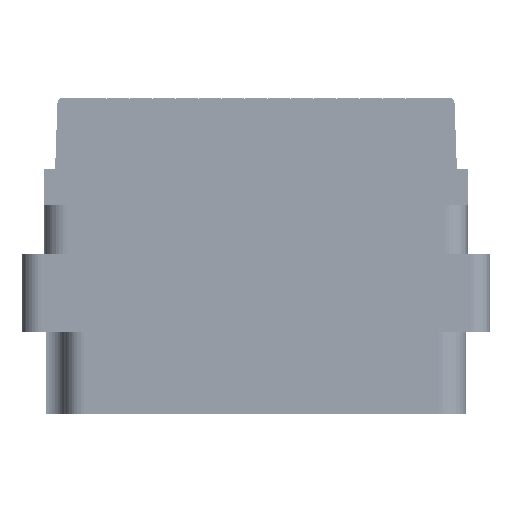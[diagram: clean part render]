
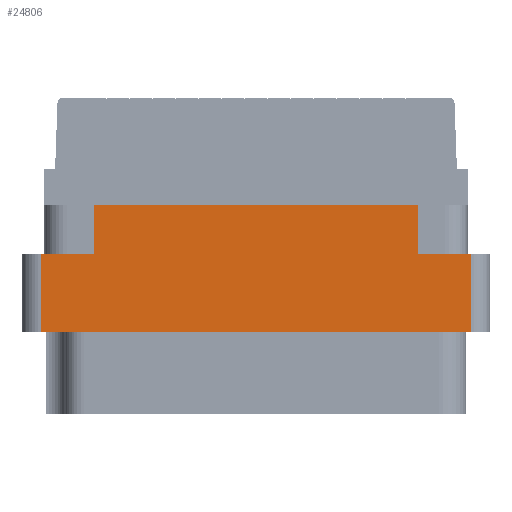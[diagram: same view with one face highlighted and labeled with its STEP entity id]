
A CAD part, left-side view. The second image highlights one B-rep face of the part: STEP entity #24806.
In plain terms, the highlighted planar face has unit normal (-1, 0, 0).
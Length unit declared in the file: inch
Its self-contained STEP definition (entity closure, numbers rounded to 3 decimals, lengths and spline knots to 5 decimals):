
#3618 = VECTOR ( 'NONE', #43353, 39.37008 ) ;
#4624 = LINE ( 'NONE', #77104, #86066 ) ;
#5512 = CARTESIAN_POINT ( 'NONE',  ( -1.375, -0.7005, -0.798 ) ) ;
#7226 = EDGE_CURVE ( 'NONE', #54643, #15740, #71783, .T. ) ;
#7428 = LINE ( 'NONE', #80379, #73741 ) ;
#8888 = AXIS2_PLACEMENT_3D ( 'NONE', #82646, #52647, #38307 ) ;
#11765 = DIRECTION ( 'NONE',  ( 0., 1., 0. ) ) ;
#11824 = VECTOR ( 'NONE', #49394, 39.37008 ) ;
#12568 = ORIENTED_EDGE ( 'NONE', *, *, #87304, .F. ) ;
#12978 = VERTEX_POINT ( 'NONE', #65259 ) ;
#13325 = CARTESIAN_POINT ( 'NONE',  ( -1.375, -0.5285, -0.277 ) ) ;
#13382 = ORIENTED_EDGE ( 'NONE', *, *, #82195, .T. ) ;
#15055 = DIRECTION ( 'NONE',  ( 0., -1., 0. ) ) ;
#15740 = VERTEX_POINT ( 'NONE', #57270 ) ;
#22085 = CARTESIAN_POINT ( 'NONE',  ( -1.375, -0.7005, -0.529 ) ) ;
#22122 = CARTESIAN_POINT ( 'NONE',  ( -1.375, 0.7625, -0.117 ) ) ;
#22387 = EDGE_CURVE ( 'NONE', #30751, #45944, #75189, .T. ) ;
#22728 = CARTESIAN_POINT ( 'NONE',  ( -1.375, 0.7005, -0.529 ) ) ;
#23524 = LINE ( 'NONE', #22122, #43030 ) ;
#24618 = DIRECTION ( 'NONE',  ( 0., 0., -1. ) ) ;
#24674 = VECTOR ( 'NONE', #59379, 39.37008 ) ;
#24806 = ADVANCED_FACE ( 'NONE', ( #39247 ), #74551, .T. ) ;
#29367 = DIRECTION ( 'NONE',  ( 0., 0., 1. ) ) ;
#30264 = LINE ( 'NONE', #60345, #24674 ) ;
#30751 = VERTEX_POINT ( 'NONE', #62207 ) ;
#31819 = VERTEX_POINT ( 'NONE', #46499 ) ;
#34468 = ORIENTED_EDGE ( 'NONE', *, *, #64064, .F. ) ;
#35543 = VERTEX_POINT ( 'NONE', #40451 ) ;
#38307 = DIRECTION ( 'NONE',  ( 0., 0., 1. ) ) ;
#39247 = FACE_OUTER_BOUND ( 'NONE', #76238, .T. ) ;
#40451 = CARTESIAN_POINT ( 'NONE',  ( -1.375, 0.5285, -0.117 ) ) ;
#43030 = VECTOR ( 'NONE', #52158, 39.37008 ) ;
#43353 = DIRECTION ( 'NONE',  ( 0., 0., 1. ) ) ;
#43817 = LINE ( 'NONE', #13325, #3618 ) ;
#45944 = VERTEX_POINT ( 'NONE', #22728 ) ;
#46499 = CARTESIAN_POINT ( 'NONE',  ( -1.375, 0.5285, -0.277 ) ) ;
#49394 = DIRECTION ( 'NONE',  ( 0., 0., 1. ) ) ;
#52158 = DIRECTION ( 'NONE',  ( 0., -1., 0. ) ) ;
#52647 = DIRECTION ( 'NONE',  ( -1., 0., 0. ) ) ;
#54196 = EDGE_CURVE ( 'NONE', #68166, #15740, #30264, .T. ) ;
#54643 = VERTEX_POINT ( 'NONE', #22085 ) ;
#57270 = CARTESIAN_POINT ( 'NONE',  ( -1.375, -0.7005, -0.277 ) ) ;
#57288 = ORIENTED_EDGE ( 'NONE', *, *, #92566, .F. ) ;
#59029 = VECTOR ( 'NONE', #29367, 39.37008 ) ;
#59379 = DIRECTION ( 'NONE',  ( 0., -1., 0. ) ) ;
#60345 = CARTESIAN_POINT ( 'NONE',  ( -1.375, 0., -0.277 ) ) ;
#62207 = CARTESIAN_POINT ( 'NONE',  ( -1.375, 0.7005, -0.277 ) ) ;
#63476 = ORIENTED_EDGE ( 'NONE', *, *, #85818, .F. ) ;
#64064 = EDGE_CURVE ( 'NONE', #54643, #45944, #4624, .T. ) ;
#65259 = CARTESIAN_POINT ( 'NONE',  ( -1.375, -0.5285, -0.117 ) ) ;
#66878 = ORIENTED_EDGE ( 'NONE', *, *, #22387, .T. ) ;
#66947 = CARTESIAN_POINT ( 'NONE',  ( -1.375, -0.5285, -0.277 ) ) ;
#68166 = VERTEX_POINT ( 'NONE', #66947 ) ;
#70281 = ORIENTED_EDGE ( 'NONE', *, *, #54196, .F. ) ;
#71783 = LINE ( 'NONE', #5512, #11824 ) ;
#72307 = VECTOR ( 'NONE', #24618, 39.37008 ) ;
#73230 = LINE ( 'NONE', #87505, #59029 ) ;
#73741 = VECTOR ( 'NONE', #15055, 39.37008 ) ;
#73875 = ORIENTED_EDGE ( 'NONE', *, *, #7226, .T. ) ;
#74551 = PLANE ( 'NONE',  #8888 ) ;
#75189 = LINE ( 'NONE', #89928, #72307 ) ;
#76238 = EDGE_LOOP ( 'NONE', ( #12568, #66878, #34468, #73875, #70281, #13382, #63476, #57288 ) ) ;
#77104 = CARTESIAN_POINT ( 'NONE',  ( -1.375, 0., -0.529 ) ) ;
#80379 = CARTESIAN_POINT ( 'NONE',  ( -1.375, 0., -0.277 ) ) ;
#82195 = EDGE_CURVE ( 'NONE', #68166, #12978, #43817, .T. ) ;
#82646 = CARTESIAN_POINT ( 'NONE',  ( -1.375, -0.7625, -0.798 ) ) ;
#85818 = EDGE_CURVE ( 'NONE', #35543, #12978, #23524, .T. ) ;
#86066 = VECTOR ( 'NONE', #11765, 39.37008 ) ;
#87304 = EDGE_CURVE ( 'NONE', #30751, #31819, #7428, .T. ) ;
#87505 = CARTESIAN_POINT ( 'NONE',  ( -1.375, 0.5285, -0.277 ) ) ;
#89928 = CARTESIAN_POINT ( 'NONE',  ( -1.375, 0.7005, -0.798 ) ) ;
#92566 = EDGE_CURVE ( 'NONE', #31819, #35543, #73230, .T. ) ;
